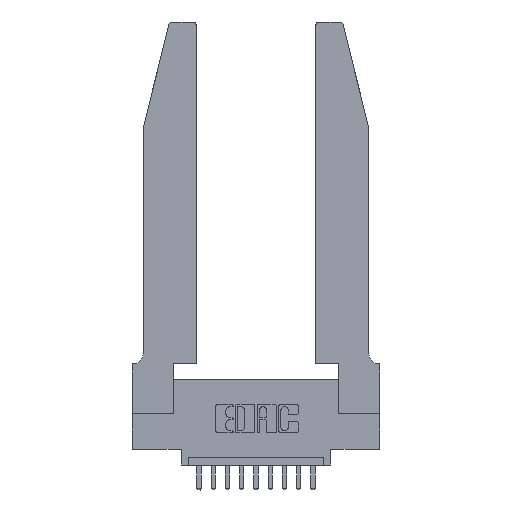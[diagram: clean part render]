
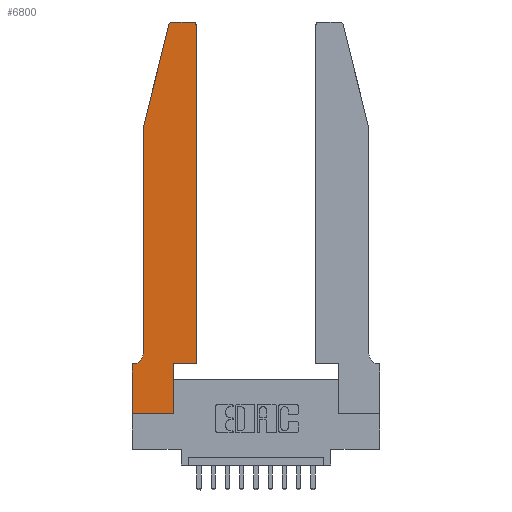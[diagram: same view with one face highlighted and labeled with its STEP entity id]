
A CAD part, top view. The second image highlights one B-rep face of the part: STEP entity #6800.
In plain terms, the highlighted planar face has unit normal (0, 0, 1).
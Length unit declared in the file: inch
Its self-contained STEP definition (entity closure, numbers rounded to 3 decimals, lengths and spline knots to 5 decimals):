
#32 = EDGE_CURVE ( 'NONE', #10940, #7605, #6862, .T. ) ;
#377 = CARTESIAN_POINT ( 'NONE',  ( 0.0755, 0.42, 0.37 ) ) ;
#525 = ORIENTED_EDGE ( 'NONE', *, *, #1771, .T. ) ;
#681 = ORIENTED_EDGE ( 'NONE', *, *, #7839, .T. ) ;
#1138 = LINE ( 'NONE', #12137, #12084 ) ;
#1524 = EDGE_CURVE ( 'NONE', #15653, #11930, #5451, .T. ) ;
#1771 = EDGE_CURVE ( 'NONE', #9702, #9956, #5052, .T. ) ;
#1831 = CARTESIAN_POINT ( 'NONE',  ( 0., 0., 0.37 ) ) ;
#2057 = CARTESIAN_POINT ( 'NONE',  ( 0., 0., 0.37 ) ) ;
#2275 = DIRECTION ( 'NONE',  ( 0., -1., 0. ) ) ;
#2387 = CARTESIAN_POINT ( 'NONE',  ( 0.4505, 0.35, 0.37 ) ) ;
#2409 = CARTESIAN_POINT ( 'NONE',  ( 0.25487, 2.72718, 0.37 ) ) ;
#2466 = DIRECTION ( 'NONE',  ( -0.239, -0.971, 0. ) ) ;
#2612 = EDGE_CURVE ( 'NONE', #9956, #10940, #11447, .T. ) ;
#2831 = DIRECTION ( 'NONE',  ( -1., 0., 0. ) ) ;
#2882 = CARTESIAN_POINT ( 'NONE',  ( 0.0055, 0.42, 0.37 ) ) ;
#2898 = DIRECTION ( 'NONE',  ( 1., 0., 0. ) ) ;
#3068 = DIRECTION ( 'NONE',  ( 0., 0., 1. ) ) ;
#3435 = VECTOR ( 'NONE', #14453, 39.37008 ) ;
#3451 = AXIS2_PLACEMENT_3D ( 'NONE', #15053, #3068, #2898 ) ;
#3583 = DIRECTION ( 'NONE',  ( 1., 0., 0. ) ) ;
#3847 = LINE ( 'NONE', #11113, #6008 ) ;
#3952 = CARTESIAN_POINT ( 'NONE',  ( 0.284, 2.72, 0.37 ) ) ;
#4128 = CARTESIAN_POINT ( 'NONE',  ( 0.0055, 0.35, 0.37 ) ) ;
#4261 = CARTESIAN_POINT ( 'NONE',  ( 0.2605, 2.75, 0.37 ) ) ;
#4610 = CARTESIAN_POINT ( 'NONE',  ( 0.0755, 2., 0.37 ) ) ;
#4726 = DIRECTION ( 'NONE',  ( 1., 0., 0. ) ) ;
#5001 = VERTEX_POINT ( 'NONE', #7948 ) ;
#5052 = LINE ( 'NONE', #12251, #14468 ) ;
#5062 = AXIS2_PLACEMENT_3D ( 'NONE', #3952, #12642, #9074 ) ;
#5160 = VECTOR ( 'NONE', #2466, 39.37008 ) ;
#5417 = CARTESIAN_POINT ( 'NONE',  ( 0.2865, 0.35, 0.37 ) ) ;
#5451 = CIRCLE ( 'NONE', #5062, 0.03 ) ;
#5468 = DIRECTION ( 'NONE',  ( 0., 0., -1. ) ) ;
#5636 = CARTESIAN_POINT ( 'NONE',  ( 0.4505, 0.35, 0.37 ) ) ;
#5967 = ORIENTED_EDGE ( 'NONE', *, *, #9047, .T. ) ;
#6008 = VECTOR ( 'NONE', #2275, 39.37008 ) ;
#6638 = ORIENTED_EDGE ( 'NONE', *, *, #15029, .T. ) ;
#6685 = VECTOR ( 'NONE', #13150, 39.37008 ) ;
#6800 = ADVANCED_FACE ( 'NONE', ( #9166 ), #12348, .T. ) ;
#6862 = LINE ( 'NONE', #2387, #13127 ) ;
#7071 = ORIENTED_EDGE ( 'NONE', *, *, #9508, .T. ) ;
#7080 = ORIENTED_EDGE ( 'NONE', *, *, #7737, .T. ) ;
#7228 = CARTESIAN_POINT ( 'NONE',  ( 0.4205, 2.72, 0.37 ) ) ;
#7413 = CARTESIAN_POINT ( 'NONE',  ( 0.2865, 0., 0.37 ) ) ;
#7530 = VERTEX_POINT ( 'NONE', #4610 ) ;
#7605 = VERTEX_POINT ( 'NONE', #14739 ) ;
#7737 = EDGE_CURVE ( 'NONE', #14809, #14849, #10304, .T. ) ;
#7839 = EDGE_CURVE ( 'NONE', #14849, #5001, #1138, .T. ) ;
#7948 = CARTESIAN_POINT ( 'NONE',  ( 0., 0.35, 0.37 ) ) ;
#8195 = CARTESIAN_POINT ( 'NONE',  ( 0.0755, 2., 0.37 ) ) ;
#8459 = AXIS2_PLACEMENT_3D ( 'NONE', #7228, #11099, #3583 ) ;
#8885 = VECTOR ( 'NONE', #15860, 39.37008 ) ;
#9047 = EDGE_CURVE ( 'NONE', #7530, #14809, #3847, .T. ) ;
#9074 = DIRECTION ( 'NONE',  ( 1., 0., 0. ) ) ;
#9166 = FACE_OUTER_BOUND ( 'NONE', #15293, .T. ) ;
#9220 = CARTESIAN_POINT ( 'NONE',  ( 0.4205, 2.75, 0.37 ) ) ;
#9440 = VERTEX_POINT ( 'NONE', #9220 ) ;
#9508 = EDGE_CURVE ( 'NONE', #9440, #15653, #10068, .T. ) ;
#9510 = AXIS2_PLACEMENT_3D ( 'NONE', #2882, #5468, #2831 ) ;
#9614 = EDGE_CURVE ( 'NONE', #5001, #13460, #15579, .T. ) ;
#9702 = VERTEX_POINT ( 'NONE', #7413 ) ;
#9812 = LINE ( 'NONE', #1831, #6685 ) ;
#9956 = VERTEX_POINT ( 'NONE', #5417 ) ;
#10068 = LINE ( 'NONE', #4261, #3435 ) ;
#10304 = CIRCLE ( 'NONE', #9510, 0.07 ) ;
#10639 = ORIENTED_EDGE ( 'NONE', *, *, #2612, .T. ) ;
#10757 = CIRCLE ( 'NONE', #8459, 0.03 ) ;
#10940 = VERTEX_POINT ( 'NONE', #5636 ) ;
#11099 = DIRECTION ( 'NONE',  ( 0., 0., 1. ) ) ;
#11113 = CARTESIAN_POINT ( 'NONE',  ( 0.0755, 2., 0.37 ) ) ;
#11157 = EDGE_CURVE ( 'NONE', #11930, #7530, #15736, .T. ) ;
#11189 = ORIENTED_EDGE ( 'NONE', *, *, #9614, .T. ) ;
#11264 = VECTOR ( 'NONE', #4726, 39.37008 ) ;
#11447 = LINE ( 'NONE', #12157, #11264 ) ;
#11930 = VERTEX_POINT ( 'NONE', #2409 ) ;
#12084 = VECTOR ( 'NONE', #15970, 39.37008 ) ;
#12137 = CARTESIAN_POINT ( 'NONE',  ( 0.0755, 0.35, 0.37 ) ) ;
#12157 = CARTESIAN_POINT ( 'NONE',  ( 0.4505, 0.35, 0.37 ) ) ;
#12243 = CARTESIAN_POINT ( 'NONE',  ( 0., 0., 0.37 ) ) ;
#12244 = EDGE_CURVE ( 'NONE', #13460, #9702, #9812, .T. ) ;
#12251 = CARTESIAN_POINT ( 'NONE',  ( 0.2865, 0.35, 0.37 ) ) ;
#12348 = PLANE ( 'NONE',  #3451 ) ;
#12642 = DIRECTION ( 'NONE',  ( 0., 0., 1. ) ) ;
#13127 = VECTOR ( 'NONE', #13672, 39.37008 ) ;
#13150 = DIRECTION ( 'NONE',  ( 1., 0., 0. ) ) ;
#13460 = VERTEX_POINT ( 'NONE', #12243 ) ;
#13672 = DIRECTION ( 'NONE',  ( 0., 1., 0. ) ) ;
#13704 = DIRECTION ( 'NONE',  ( 0., 1., 0. ) ) ;
#14453 = DIRECTION ( 'NONE',  ( -1., 0., 0. ) ) ;
#14468 = VECTOR ( 'NONE', #13704, 39.37008 ) ;
#14635 = ORIENTED_EDGE ( 'NONE', *, *, #32, .T. ) ;
#14739 = CARTESIAN_POINT ( 'NONE',  ( 0.4505, 2.72, 0.37 ) ) ;
#14745 = ORIENTED_EDGE ( 'NONE', *, *, #12244, .T. ) ;
#14809 = VERTEX_POINT ( 'NONE', #377 ) ;
#14845 = CARTESIAN_POINT ( 'NONE',  ( 0.284, 2.75, 0.37 ) ) ;
#14849 = VERTEX_POINT ( 'NONE', #4128 ) ;
#15029 = EDGE_CURVE ( 'NONE', #7605, #9440, #10757, .T. ) ;
#15053 = CARTESIAN_POINT ( 'NONE',  ( 0., 0.35, 0.37 ) ) ;
#15293 = EDGE_LOOP ( 'NONE', ( #7071, #15676, #16056, #5967, #7080, #681, #11189, #14745, #525, #10639, #14635, #6638 ) ) ;
#15579 = LINE ( 'NONE', #2057, #8885 ) ;
#15653 = VERTEX_POINT ( 'NONE', #14845 ) ;
#15676 = ORIENTED_EDGE ( 'NONE', *, *, #1524, .T. ) ;
#15736 = LINE ( 'NONE', #8195, #5160 ) ;
#15860 = DIRECTION ( 'NONE',  ( 0., -1., 0. ) ) ;
#15970 = DIRECTION ( 'NONE',  ( -1., 0., 0. ) ) ;
#16056 = ORIENTED_EDGE ( 'NONE', *, *, #11157, .T. ) ;
